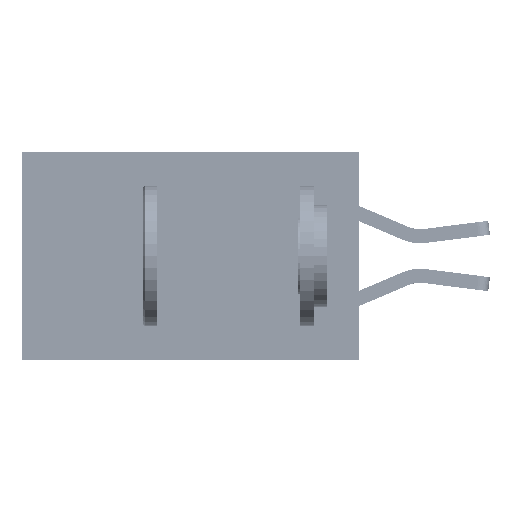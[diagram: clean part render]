
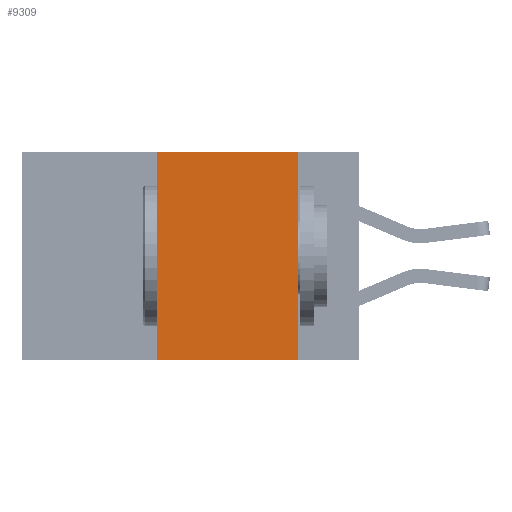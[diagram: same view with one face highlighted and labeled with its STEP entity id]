
A CAD part, left-side view. The second image highlights one B-rep face of the part: STEP entity #9309.
In plain terms, the highlighted planar face has unit normal (-1, 0, 0).
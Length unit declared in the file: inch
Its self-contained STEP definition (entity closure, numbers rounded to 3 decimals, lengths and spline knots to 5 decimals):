
#5164 = DIRECTION ( 'NONE',  ( 1., 0., 0. ) ) ;
#6061 = CARTESIAN_POINT ( 'NONE',  ( 0., 0.11, -0.37 ) ) ;
#8772 = CARTESIAN_POINT ( 'NONE',  ( 0., 0.11, 0. ) ) ;
#9309 = ADVANCED_FACE ( 'NONE', ( #41673 ), #41169, .F. ) ;
#10830 = ORIENTED_EDGE ( 'NONE', *, *, #24042, .F. ) ;
#11841 = EDGE_CURVE ( 'NONE', #40620, #27360, #38380, .T. ) ;
#12340 = CARTESIAN_POINT ( 'NONE',  ( 0., 0.11, 0. ) ) ;
#14160 = DIRECTION ( 'NONE',  ( 0., -1., 0. ) ) ;
#16086 = CARTESIAN_POINT ( 'NONE',  ( 0., 0.36, 0. ) ) ;
#16275 = CARTESIAN_POINT ( 'NONE',  ( 0., 0.6, 0. ) ) ;
#16296 = DIRECTION ( 'NONE',  ( 0., 0., -1. ) ) ;
#17860 = DIRECTION ( 'NONE',  ( 0., -1., 0. ) ) ;
#19849 = DIRECTION ( 'NONE',  ( 0., 0., 1. ) ) ;
#20237 = VERTEX_POINT ( 'NONE', #44873 ) ;
#22487 = EDGE_LOOP ( 'NONE', ( #46401, #39696, #10830, #23632 ) ) ;
#23601 = VECTOR ( 'NONE', #16296, 39.37008 ) ;
#23632 = ORIENTED_EDGE ( 'NONE', *, *, #34791, .T. ) ;
#24042 = EDGE_CURVE ( 'NONE', #20237, #40620, #36640, .T. ) ;
#24321 = VECTOR ( 'NONE', #19849, 39.37008 ) ;
#27257 = VECTOR ( 'NONE', #14160, 39.37008 ) ;
#27360 = VERTEX_POINT ( 'NONE', #12340 ) ;
#27427 = VERTEX_POINT ( 'NONE', #6061 ) ;
#34791 = EDGE_CURVE ( 'NONE', #20237, #27427, #37152, .T. ) ;
#35879 = LINE ( 'NONE', #8772, #23601 ) ;
#36225 = CARTESIAN_POINT ( 'NONE',  ( 0., 0.36, 0. ) ) ;
#36227 = CARTESIAN_POINT ( 'NONE',  ( 0., 0.6, -0.37 ) ) ;
#36640 = LINE ( 'NONE', #16086, #24321 ) ;
#37152 = LINE ( 'NONE', #36227, #45520 ) ;
#37753 = DIRECTION ( 'NONE',  ( 0., 0., -1. ) ) ;
#37771 = EDGE_CURVE ( 'NONE', #27360, #27427, #35879, .T. ) ;
#38380 = LINE ( 'NONE', #42533, #27257 ) ;
#39696 = ORIENTED_EDGE ( 'NONE', *, *, #11841, .F. ) ;
#40590 = AXIS2_PLACEMENT_3D ( 'NONE', #16275, #5164, #37753 ) ;
#40620 = VERTEX_POINT ( 'NONE', #36225 ) ;
#41169 = PLANE ( 'NONE',  #40590 ) ;
#41673 = FACE_OUTER_BOUND ( 'NONE', #22487, .T. ) ;
#42533 = CARTESIAN_POINT ( 'NONE',  ( 0., 0.6, 0. ) ) ;
#44873 = CARTESIAN_POINT ( 'NONE',  ( 0., 0.36, -0.37 ) ) ;
#45520 = VECTOR ( 'NONE', #17860, 39.37008 ) ;
#46401 = ORIENTED_EDGE ( 'NONE', *, *, #37771, .F. ) ;
